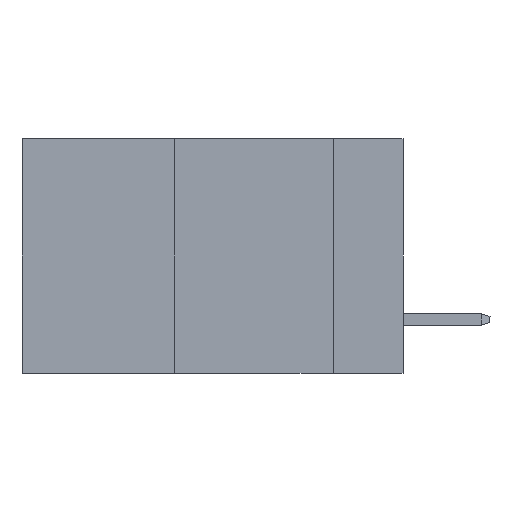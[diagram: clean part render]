
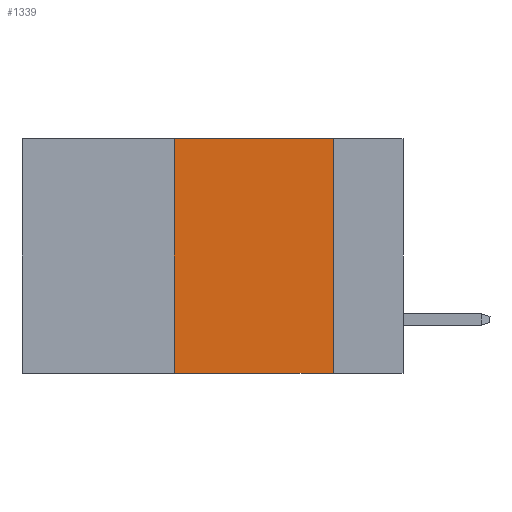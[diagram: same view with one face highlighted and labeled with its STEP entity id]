
A CAD part, left-side view. The second image highlights one B-rep face of the part: STEP entity #1339.
In plain terms, the highlighted planar face has unit normal (-1, 0, 0).
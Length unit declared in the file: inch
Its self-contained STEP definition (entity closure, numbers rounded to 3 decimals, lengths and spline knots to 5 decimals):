
#52 = PLANE ( 'NONE',  #801 ) ;
#248 = CARTESIAN_POINT ( 'NONE',  ( 0., 0.11, 0. ) ) ;
#602 = VECTOR ( 'NONE', #7543, 39.37008 ) ;
#636 = LINE ( 'NONE', #5538, #602 ) ;
#651 = DIRECTION ( 'NONE',  ( 0., -1., 0. ) ) ;
#801 = AXIS2_PLACEMENT_3D ( 'NONE', #6293, #8236, #6257 ) ;
#968 = LINE ( 'NONE', #248, #5525 ) ;
#1276 = CARTESIAN_POINT ( 'NONE',  ( 0., 0.11, 0. ) ) ;
#1339 = ADVANCED_FACE ( 'NONE', ( #3539 ), #52, .F. ) ;
#1381 = CARTESIAN_POINT ( 'NONE',  ( 0., 0.6, -0.37 ) ) ;
#1659 = VERTEX_POINT ( 'NONE', #1276 ) ;
#1959 = VERTEX_POINT ( 'NONE', #5519 ) ;
#2530 = EDGE_LOOP ( 'NONE', ( #7845, #7023, #7443, #6602 ) ) ;
#2869 = VECTOR ( 'NONE', #651, 39.37008 ) ;
#2955 = EDGE_CURVE ( 'NONE', #4116, #1959, #7695, .T. ) ;
#3539 = FACE_OUTER_BOUND ( 'NONE', #2530, .T. ) ;
#4116 = VERTEX_POINT ( 'NONE', #8171 ) ;
#4418 = DIRECTION ( 'NONE',  ( 0., 0., -1. ) ) ;
#4619 = LINE ( 'NONE', #7433, #6089 ) ;
#5519 = CARTESIAN_POINT ( 'NONE',  ( 0., 0.11, -0.37 ) ) ;
#5525 = VECTOR ( 'NONE', #4418, 39.37008 ) ;
#5538 = CARTESIAN_POINT ( 'NONE',  ( 0., 0.6, 0. ) ) ;
#5705 = EDGE_CURVE ( 'NONE', #4116, #6808, #4619, .T. ) ;
#6089 = VECTOR ( 'NONE', #7354, 39.37008 ) ;
#6257 = DIRECTION ( 'NONE',  ( 0., 0., -1. ) ) ;
#6293 = CARTESIAN_POINT ( 'NONE',  ( 0., 0.6, 0. ) ) ;
#6602 = ORIENTED_EDGE ( 'NONE', *, *, #2955, .T. ) ;
#6808 = VERTEX_POINT ( 'NONE', #7436 ) ;
#6963 = EDGE_CURVE ( 'NONE', #1659, #1959, #968, .T. ) ;
#7023 = ORIENTED_EDGE ( 'NONE', *, *, #7248, .F. ) ;
#7248 = EDGE_CURVE ( 'NONE', #6808, #1659, #636, .T. ) ;
#7354 = DIRECTION ( 'NONE',  ( 0., 0., 1. ) ) ;
#7433 = CARTESIAN_POINT ( 'NONE',  ( 0., 0.36, 0. ) ) ;
#7436 = CARTESIAN_POINT ( 'NONE',  ( 0., 0.36, 0. ) ) ;
#7443 = ORIENTED_EDGE ( 'NONE', *, *, #5705, .F. ) ;
#7543 = DIRECTION ( 'NONE',  ( 0., -1., 0. ) ) ;
#7695 = LINE ( 'NONE', #1381, #2869 ) ;
#7845 = ORIENTED_EDGE ( 'NONE', *, *, #6963, .F. ) ;
#8171 = CARTESIAN_POINT ( 'NONE',  ( 0., 0.36, -0.37 ) ) ;
#8236 = DIRECTION ( 'NONE',  ( 1., 0., 0. ) ) ;
